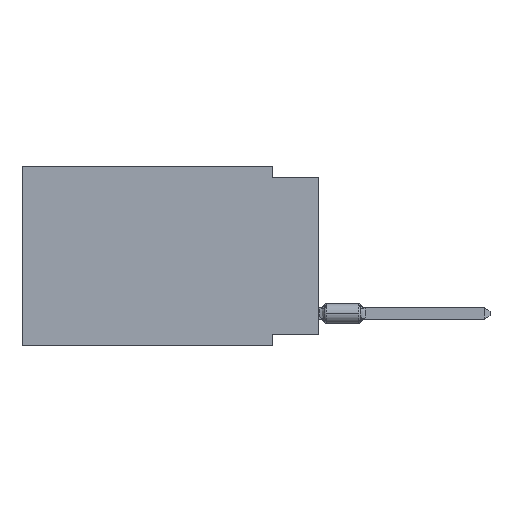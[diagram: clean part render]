
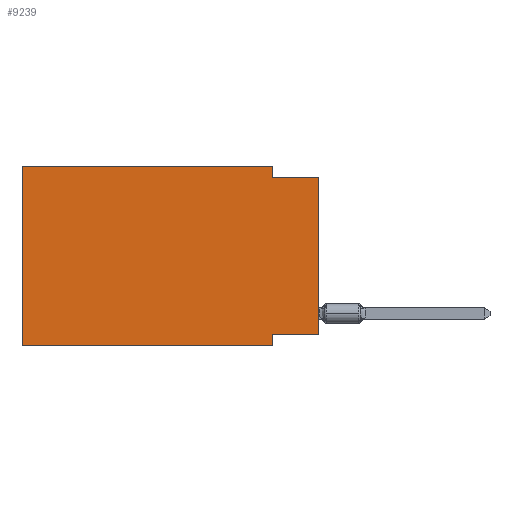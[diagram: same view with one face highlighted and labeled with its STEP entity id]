
A CAD part, left-side view. The second image highlights one B-rep face of the part: STEP entity #9239.
In plain terms, the highlighted planar face has unit normal (-1, 0, 0).
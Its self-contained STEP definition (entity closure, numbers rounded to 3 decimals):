
#275 = ORIENTED_EDGE ( 'NONE', *, *, #6059, .T. ) ;
#952 = VECTOR ( 'NONE', #13263, 1000. ) ;
#1027 = VERTEX_POINT ( 'NONE', #6702 ) ;
#1266 = LINE ( 'NONE', #2928, #10971 ) ;
#1493 = DIRECTION ( 'NONE',  ( 0., 0., 1. ) ) ;
#2667 = VERTEX_POINT ( 'NONE', #5865 ) ;
#2787 = EDGE_CURVE ( 'NONE', #1027, #16025, #12246, .T. ) ;
#2838 = DIRECTION ( 'NONE',  ( 0., -1., 0. ) ) ;
#2842 = VECTOR ( 'NONE', #17114, 1000. ) ;
#2928 = CARTESIAN_POINT ( 'NONE',  ( 0., 0., -0.635 ) ) ;
#3067 = VECTOR ( 'NONE', #8017, 1000. ) ;
#3288 = ORIENTED_EDGE ( 'NONE', *, *, #7664, .F. ) ;
#3711 = VECTOR ( 'NONE', #17581, 1000. ) ;
#3944 = VECTOR ( 'NONE', #1493, 1000. ) ;
#4419 = VECTOR ( 'NONE', #10741, 1000. ) ;
#4727 = ORIENTED_EDGE ( 'NONE', *, *, #2787, .F. ) ;
#4855 = CARTESIAN_POINT ( 'NONE',  ( 0., 16.383, 0. ) ) ;
#5201 = ORIENTED_EDGE ( 'NONE', *, *, #10579, .F. ) ;
#5564 = CARTESIAN_POINT ( 'NONE',  ( 0., 2.54, -9.271 ) ) ;
#5724 = ORIENTED_EDGE ( 'NONE', *, *, #9633, .T. ) ;
#5865 = CARTESIAN_POINT ( 'NONE',  ( 0., 0., -0.635 ) ) ;
#6059 = EDGE_CURVE ( 'NONE', #17042, #2667, #17010, .T. ) ;
#6473 = ORIENTED_EDGE ( 'NONE', *, *, #9035, .F. ) ;
#6702 = CARTESIAN_POINT ( 'NONE',  ( 0., 16.383, -9.906 ) ) ;
#6825 = VERTEX_POINT ( 'NONE', #5564 ) ;
#7078 = EDGE_CURVE ( 'NONE', #16025, #17318, #16022, .T. ) ;
#7664 = EDGE_CURVE ( 'NONE', #17042, #6825, #8445, .T. ) ;
#8017 = DIRECTION ( 'NONE',  ( 0., 0., 1. ) ) ;
#8445 = LINE ( 'NONE', #12771, #2842 ) ;
#8541 = CARTESIAN_POINT ( 'NONE',  ( 0., 16.383, 0. ) ) ;
#9035 = EDGE_CURVE ( 'NONE', #6825, #13121, #15953, .T. ) ;
#9182 = CARTESIAN_POINT ( 'NONE',  ( 0., 2.54, -9.906 ) ) ;
#9239 = ADVANCED_FACE ( 'NONE', ( #16839 ), #11303, .F. ) ;
#9633 = EDGE_CURVE ( 'NONE', #1027, #13121, #15348, .T. ) ;
#9990 = CARTESIAN_POINT ( 'NONE',  ( 0., 0., 0. ) ) ;
#10541 = ORIENTED_EDGE ( 'NONE', *, *, #14194, .F. ) ;
#10579 = EDGE_CURVE ( 'NONE', #17318, #15816, #12126, .T. ) ;
#10741 = DIRECTION ( 'NONE',  ( 0., 0., -1. ) ) ;
#10971 = VECTOR ( 'NONE', #2838, 1000. ) ;
#11041 = CARTESIAN_POINT ( 'NONE',  ( 0., 2.54, -0.635 ) ) ;
#11303 = PLANE ( 'NONE',  #12449 ) ;
#12126 = LINE ( 'NONE', #17753, #4419 ) ;
#12246 = LINE ( 'NONE', #13277, #3067 ) ;
#12449 = AXIS2_PLACEMENT_3D ( 'NONE', #8541, #17118, #17031 ) ;
#12666 = CARTESIAN_POINT ( 'NONE',  ( 0., 16.383, -9.906 ) ) ;
#12771 = CARTESIAN_POINT ( 'NONE',  ( 0., 0., -9.271 ) ) ;
#13121 = VERTEX_POINT ( 'NONE', #9182 ) ;
#13263 = DIRECTION ( 'NONE',  ( 0., 0., -1. ) ) ;
#13277 = CARTESIAN_POINT ( 'NONE',  ( 0., 16.383, 0. ) ) ;
#13338 = ORIENTED_EDGE ( 'NONE', *, *, #7078, .F. ) ;
#14194 = EDGE_CURVE ( 'NONE', #15816, #2667, #1266, .T. ) ;
#14743 = CARTESIAN_POINT ( 'NONE',  ( 0., 2.54, -9.906 ) ) ;
#14907 = CARTESIAN_POINT ( 'NONE',  ( 0., 16.383, 0. ) ) ;
#15348 = LINE ( 'NONE', #12666, #15372 ) ;
#15372 = VECTOR ( 'NONE', #18114, 1000. ) ;
#15816 = VERTEX_POINT ( 'NONE', #11041 ) ;
#15953 = LINE ( 'NONE', #14743, #952 ) ;
#16022 = LINE ( 'NONE', #14907, #3711 ) ;
#16025 = VERTEX_POINT ( 'NONE', #4855 ) ;
#16523 = CARTESIAN_POINT ( 'NONE',  ( 0., 2.54, 0. ) ) ;
#16839 = FACE_OUTER_BOUND ( 'NONE', #17257, .T. ) ;
#17010 = LINE ( 'NONE', #9990, #3944 ) ;
#17031 = DIRECTION ( 'NONE',  ( 0., 0., -1. ) ) ;
#17042 = VERTEX_POINT ( 'NONE', #18034 ) ;
#17114 = DIRECTION ( 'NONE',  ( 0., 1., 0. ) ) ;
#17118 = DIRECTION ( 'NONE',  ( 1., 0., 0. ) ) ;
#17257 = EDGE_LOOP ( 'NONE', ( #275, #10541, #5201, #13338, #4727, #5724, #6473, #3288 ) ) ;
#17318 = VERTEX_POINT ( 'NONE', #16523 ) ;
#17581 = DIRECTION ( 'NONE',  ( 0., -1., 0. ) ) ;
#17753 = CARTESIAN_POINT ( 'NONE',  ( 0., 2.54, 0. ) ) ;
#18034 = CARTESIAN_POINT ( 'NONE',  ( 0., 0., -9.271 ) ) ;
#18114 = DIRECTION ( 'NONE',  ( 0., -1., 0. ) ) ;
